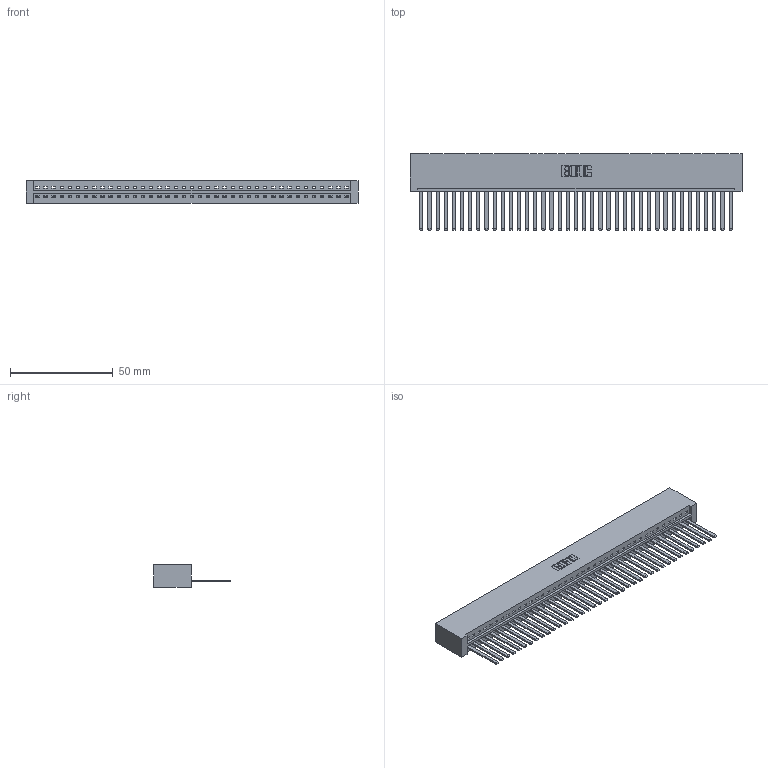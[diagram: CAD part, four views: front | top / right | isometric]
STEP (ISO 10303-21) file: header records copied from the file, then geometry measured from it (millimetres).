
FILE_DESCRIPTION (( 'STEP AP203' ), '1' );
FILE_NAME ('336-039-541-601.STEP', '2020-08-07T23:08:18', ( '' ), ( '' ), 'SwSTEP 2.0', 'SolidWorks 2020', '' );
FILE_SCHEMA (( 'CONFIG_CONTROL_DESIGN' ));
Length unit declared in the file: inch
Products named in the file (3): 336-290-001_336-290-541; 336 Part_Lugless; 336-039-541-601
Assembly tree (40 placements, depth 2):
  336-039-541-601
    336 Part_Lugless
    336-290-001_336-290-541  x39
Bounding box: 161.65 x 37.34 x 11.1 mm (x, y, z)
Volume: 25001.2 mm3; surface area: 27208.8 mm2
Topology: 40 solids, 40 shells, 2056 faces, 6293 edges, 4168 vertices
Faces by surface type: plane 1392, cylinder 664
Entity records: 28820 total; most frequent: CARTESIAN_POINT 5110, ORIENTED_EDGE 4986, DIRECTION 4203, EDGE_CURVE 2493, LINE 2369, VECTOR 2369, VERTEX_POINT 1660, AXIS2_PLACEMENT_3D 917
